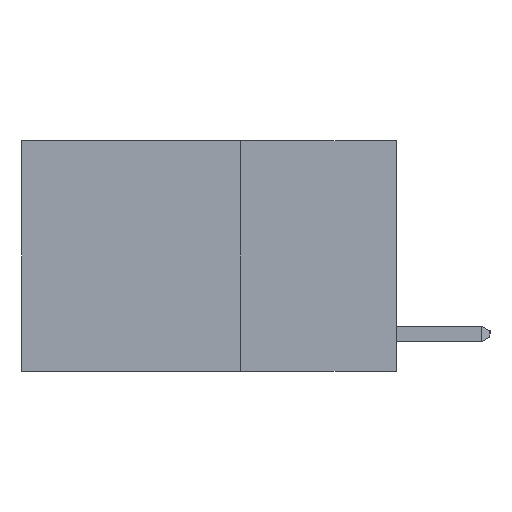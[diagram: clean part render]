
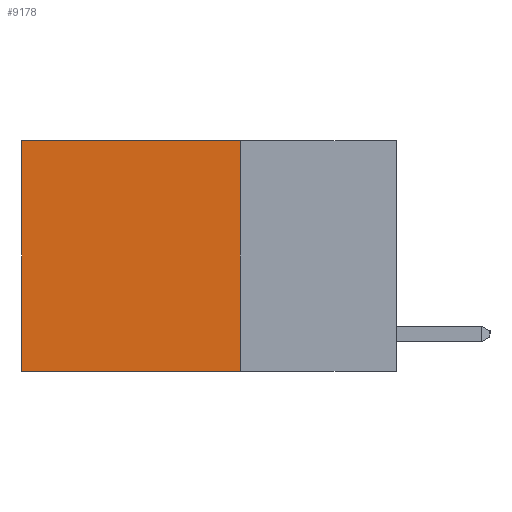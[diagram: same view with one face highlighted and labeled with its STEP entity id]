
A CAD part, left-side view. The second image highlights one B-rep face of the part: STEP entity #9178.
In plain terms, the highlighted planar face has unit normal (-1, 0, 0).
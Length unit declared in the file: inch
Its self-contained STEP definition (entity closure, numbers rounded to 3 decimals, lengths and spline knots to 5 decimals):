
#502 = VECTOR ( 'NONE', #15558, 39.37008 ) ;
#549 = VERTEX_POINT ( 'NONE', #13239 ) ;
#1122 = LINE ( 'NONE', #15202, #4160 ) ;
#1448 = CARTESIAN_POINT ( 'NONE',  ( 0.2625, 0.25, 0. ) ) ;
#1788 = EDGE_CURVE ( 'NONE', #549, #4080, #3922, .T. ) ;
#2029 = ORIENTED_EDGE ( 'NONE', *, *, #2140, .T. ) ;
#2140 = EDGE_CURVE ( 'NONE', #14192, #549, #14755, .T. ) ;
#2756 = DIRECTION ( 'NONE',  ( 1., 0., 0. ) ) ;
#2760 = CARTESIAN_POINT ( 'NONE',  ( 0.2625, 0.6, 0. ) ) ;
#3402 = EDGE_CURVE ( 'NONE', #3910, #4080, #9933, .T. ) ;
#3910 = VERTEX_POINT ( 'NONE', #13298 ) ;
#3922 = LINE ( 'NONE', #2760, #502 ) ;
#4080 = VERTEX_POINT ( 'NONE', #11175 ) ;
#4160 = VECTOR ( 'NONE', #6905, 39.37008 ) ;
#6681 = VECTOR ( 'NONE', #7566, 39.37008 ) ;
#6905 = DIRECTION ( 'NONE',  ( 0., 0., -1. ) ) ;
#7554 = EDGE_LOOP ( 'NONE', ( #11192, #14323, #8423, #2029 ) ) ;
#7566 = DIRECTION ( 'NONE',  ( 0., 1., 0. ) ) ;
#8423 = ORIENTED_EDGE ( 'NONE', *, *, #11623, .F. ) ;
#9091 = PLANE ( 'NONE',  #11138 ) ;
#9178 = ADVANCED_FACE ( 'NONE', ( #13176 ), #9091, .F. ) ;
#9933 = LINE ( 'NONE', #14685, #6681 ) ;
#11037 = CARTESIAN_POINT ( 'NONE',  ( 0.2625, 0.25, 0. ) ) ;
#11138 = AXIS2_PLACEMENT_3D ( 'NONE', #1448, #2756, #11441 ) ;
#11175 = CARTESIAN_POINT ( 'NONE',  ( 0.2625, 0.6, -0.37 ) ) ;
#11192 = ORIENTED_EDGE ( 'NONE', *, *, #1788, .T. ) ;
#11441 = DIRECTION ( 'NONE',  ( 0., 0., -1. ) ) ;
#11623 = EDGE_CURVE ( 'NONE', #14192, #3910, #1122, .T. ) ;
#11631 = VECTOR ( 'NONE', #12593, 39.37008 ) ;
#12593 = DIRECTION ( 'NONE',  ( 0., 1., 0. ) ) ;
#13176 = FACE_OUTER_BOUND ( 'NONE', #7554, .T. ) ;
#13239 = CARTESIAN_POINT ( 'NONE',  ( 0.2625, 0.6, 0. ) ) ;
#13298 = CARTESIAN_POINT ( 'NONE',  ( 0.2625, 0.25, -0.37 ) ) ;
#13400 = CARTESIAN_POINT ( 'NONE',  ( 0.2625, 0.25, 0. ) ) ;
#14192 = VERTEX_POINT ( 'NONE', #11037 ) ;
#14323 = ORIENTED_EDGE ( 'NONE', *, *, #3402, .F. ) ;
#14685 = CARTESIAN_POINT ( 'NONE',  ( 0.2625, 0.25, -0.37 ) ) ;
#14755 = LINE ( 'NONE', #13400, #11631 ) ;
#15202 = CARTESIAN_POINT ( 'NONE',  ( 0.2625, 0.25, 0. ) ) ;
#15558 = DIRECTION ( 'NONE',  ( 0., 0., -1. ) ) ;
